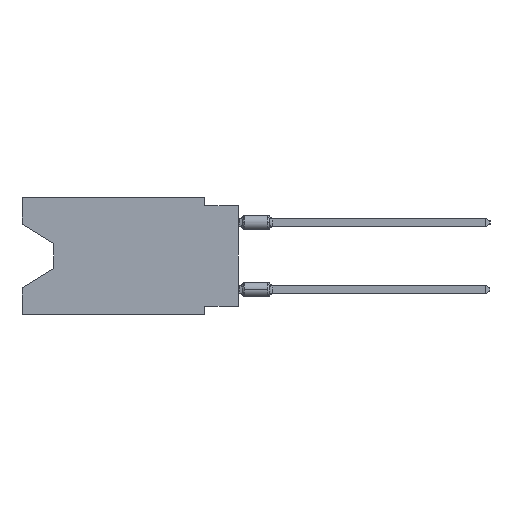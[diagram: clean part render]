
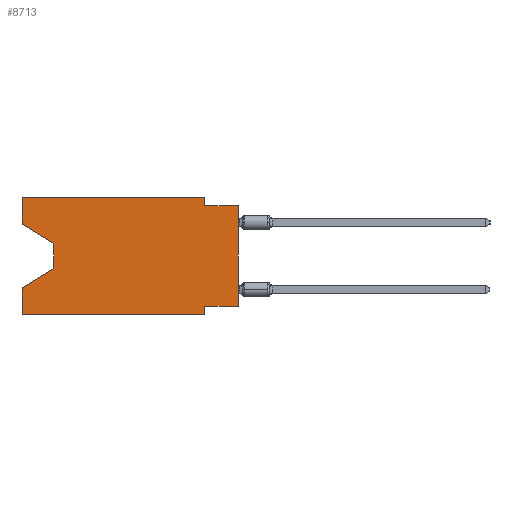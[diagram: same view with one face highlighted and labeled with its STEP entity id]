
A CAD part, left-side view. The second image highlights one B-rep face of the part: STEP entity #8713.
In plain terms, the highlighted planar face has unit normal (-1, 0, 0).
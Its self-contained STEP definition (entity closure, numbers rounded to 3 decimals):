
#262 = VECTOR ( 'NONE', #4472, 1000. ) ;
#289 = LINE ( 'NONE', #21041, #15894 ) ;
#421 = ORIENTED_EDGE ( 'NONE', *, *, #34585, .F. ) ;
#763 = EDGE_CURVE ( 'NONE', #27127, #10807, #26674, .T. ) ;
#1056 = DIRECTION ( 'NONE',  ( 0., -1., 0. ) ) ;
#1102 = CARTESIAN_POINT ( 'NONE',  ( 0., 16.383, -2.038 ) ) ;
#1876 = LINE ( 'NONE', #37017, #10331 ) ;
#2037 = LINE ( 'NONE', #4490, #2582 ) ;
#2582 = VECTOR ( 'NONE', #8059, 1000. ) ;
#3258 = VERTEX_POINT ( 'NONE', #36869 ) ;
#4444 = DIRECTION ( 'NONE',  ( 0., 0., 1. ) ) ;
#4472 = DIRECTION ( 'NONE',  ( 0., 0., -1. ) ) ;
#4490 = CARTESIAN_POINT ( 'NONE',  ( 0., 0., -0.635 ) ) ;
#5531 = CARTESIAN_POINT ( 'NONE',  ( 0., 16.383, -6.852 ) ) ;
#6348 = CARTESIAN_POINT ( 'NONE',  ( 0., 16.383, -8.89 ) ) ;
#6376 = DIRECTION ( 'NONE',  ( 1., 0., 0. ) ) ;
#7094 = LINE ( 'NONE', #15231, #14601 ) ;
#7292 = CARTESIAN_POINT ( 'NONE',  ( 0., 2.54, -8.89 ) ) ;
#7312 = CARTESIAN_POINT ( 'NONE',  ( 0., 13.97, -5.385 ) ) ;
#8059 = DIRECTION ( 'NONE',  ( 0., -1., 0. ) ) ;
#8412 = VERTEX_POINT ( 'NONE', #35254 ) ;
#8562 = VECTOR ( 'NONE', #34032, 1000. ) ;
#8713 = ADVANCED_FACE ( 'NONE', ( #29999 ), #35109, .F. ) ;
#9758 = DIRECTION ( 'NONE',  ( 0., 0., -1. ) ) ;
#9831 = VECTOR ( 'NONE', #27547, 1000. ) ;
#9863 = CARTESIAN_POINT ( 'NONE',  ( 0., 2.54, -8.89 ) ) ;
#10045 = ORIENTED_EDGE ( 'NONE', *, *, #763, .F. ) ;
#10190 = DIRECTION ( 'NONE',  ( 0., 0., 1. ) ) ;
#10331 = VECTOR ( 'NONE', #34185, 1000. ) ;
#10807 = VERTEX_POINT ( 'NONE', #35872 ) ;
#10969 = LINE ( 'NONE', #25162, #8562 ) ;
#11024 = VERTEX_POINT ( 'NONE', #36984 ) ;
#12344 = DIRECTION ( 'NONE',  ( 0., -1., 0. ) ) ;
#13097 = EDGE_CURVE ( 'NONE', #30204, #28272, #15877, .T. ) ;
#13838 = EDGE_CURVE ( 'NONE', #23940, #8412, #7094, .T. ) ;
#13853 = CARTESIAN_POINT ( 'NONE',  ( 0., 2.54, -8.255 ) ) ;
#14453 = CARTESIAN_POINT ( 'NONE',  ( 0., 0., -8.255 ) ) ;
#14601 = VECTOR ( 'NONE', #4444, 1000. ) ;
#15020 = EDGE_LOOP ( 'NONE', ( #34271, #21767, #30359, #18782, #26481, #421, #30838, #36578, #17789, #37287, #33578, #10045 ) ) ;
#15231 = CARTESIAN_POINT ( 'NONE',  ( 0., 0., 0. ) ) ;
#15499 = EDGE_CURVE ( 'NONE', #30204, #25587, #23366, .T. ) ;
#15877 = LINE ( 'NONE', #27414, #19702 ) ;
#15894 = VECTOR ( 'NONE', #12344, 1000. ) ;
#17789 = ORIENTED_EDGE ( 'NONE', *, *, #19752, .F. ) ;
#18639 = VECTOR ( 'NONE', #1056, 1000. ) ;
#18657 = CARTESIAN_POINT ( 'NONE',  ( 0., 16.383, -8.89 ) ) ;
#18782 = ORIENTED_EDGE ( 'NONE', *, *, #13097, .F. ) ;
#19695 = VERTEX_POINT ( 'NONE', #7312 ) ;
#19702 = VECTOR ( 'NONE', #10190, 1000. ) ;
#19752 = EDGE_CURVE ( 'NONE', #11024, #8412, #2037, .T. ) ;
#20224 = VERTEX_POINT ( 'NONE', #27878 ) ;
#20374 = EDGE_CURVE ( 'NONE', #10807, #20224, #289, .T. ) ;
#20463 = VECTOR ( 'NONE', #24564, 1000. ) ;
#21041 = CARTESIAN_POINT ( 'NONE',  ( 0., 16.383, 0. ) ) ;
#21767 = ORIENTED_EDGE ( 'NONE', *, *, #29984, .T. ) ;
#22931 = LINE ( 'NONE', #23496, #25750 ) ;
#23366 = LINE ( 'NONE', #6348, #18639 ) ;
#23496 = CARTESIAN_POINT ( 'NONE',  ( 0., 2.54, 0. ) ) ;
#23940 = VERTEX_POINT ( 'NONE', #14453 ) ;
#24007 = CARTESIAN_POINT ( 'NONE',  ( 0., 16.383, 0. ) ) ;
#24564 = DIRECTION ( 'NONE',  ( 0., 0., 1. ) ) ;
#25162 = CARTESIAN_POINT ( 'NONE',  ( 0., 13.97, -3.505 ) ) ;
#25458 = EDGE_CURVE ( 'NONE', #20224, #11024, #22931, .T. ) ;
#25587 = VERTEX_POINT ( 'NONE', #9863 ) ;
#25750 = VECTOR ( 'NONE', #34850, 1000. ) ;
#26481 = ORIENTED_EDGE ( 'NONE', *, *, #15499, .T. ) ;
#26627 = DIRECTION ( 'NONE',  ( 0., -0.855, -0.519 ) ) ;
#26674 = LINE ( 'NONE', #24007, #20463 ) ;
#26998 = LINE ( 'NONE', #1102, #36979 ) ;
#27127 = VERTEX_POINT ( 'NONE', #34210 ) ;
#27414 = CARTESIAN_POINT ( 'NONE',  ( 0., 16.383, 0. ) ) ;
#27547 = DIRECTION ( 'NONE',  ( 0., 1., 0. ) ) ;
#27878 = CARTESIAN_POINT ( 'NONE',  ( 0., 2.54, 0. ) ) ;
#28272 = VERTEX_POINT ( 'NONE', #5531 ) ;
#29258 = CARTESIAN_POINT ( 'NONE',  ( 0., 16.383, 0. ) ) ;
#29984 = EDGE_CURVE ( 'NONE', #3258, #19695, #10969, .T. ) ;
#29999 = FACE_OUTER_BOUND ( 'NONE', #15020, .T. ) ;
#30182 = LINE ( 'NONE', #7292, #262 ) ;
#30204 = VERTEX_POINT ( 'NONE', #18657 ) ;
#30359 = ORIENTED_EDGE ( 'NONE', *, *, #35945, .T. ) ;
#30838 = ORIENTED_EDGE ( 'NONE', *, *, #33703, .F. ) ;
#31153 = VERTEX_POINT ( 'NONE', #13853 ) ;
#33437 = AXIS2_PLACEMENT_3D ( 'NONE', #29258, #6376, #9758 ) ;
#33578 = ORIENTED_EDGE ( 'NONE', *, *, #20374, .F. ) ;
#33622 = EDGE_CURVE ( 'NONE', #27127, #3258, #26998, .T. ) ;
#33703 = EDGE_CURVE ( 'NONE', #23940, #31153, #36051, .T. ) ;
#34032 = DIRECTION ( 'NONE',  ( 0., 0., -1. ) ) ;
#34185 = DIRECTION ( 'NONE',  ( 0., 0.855, -0.519 ) ) ;
#34210 = CARTESIAN_POINT ( 'NONE',  ( 0., 16.383, -2.038 ) ) ;
#34271 = ORIENTED_EDGE ( 'NONE', *, *, #33622, .T. ) ;
#34585 = EDGE_CURVE ( 'NONE', #31153, #25587, #30182, .T. ) ;
#34850 = DIRECTION ( 'NONE',  ( 0., 0., -1. ) ) ;
#35109 = PLANE ( 'NONE',  #33437 ) ;
#35254 = CARTESIAN_POINT ( 'NONE',  ( 0., 0., -0.635 ) ) ;
#35872 = CARTESIAN_POINT ( 'NONE',  ( 0., 16.383, 0. ) ) ;
#35945 = EDGE_CURVE ( 'NONE', #19695, #28272, #1876, .T. ) ;
#36051 = LINE ( 'NONE', #36420, #9831 ) ;
#36420 = CARTESIAN_POINT ( 'NONE',  ( 0., 0., -8.255 ) ) ;
#36578 = ORIENTED_EDGE ( 'NONE', *, *, #13838, .T. ) ;
#36869 = CARTESIAN_POINT ( 'NONE',  ( 0., 13.97, -3.505 ) ) ;
#36979 = VECTOR ( 'NONE', #26627, 1000. ) ;
#36984 = CARTESIAN_POINT ( 'NONE',  ( 0., 2.54, -0.635 ) ) ;
#37017 = CARTESIAN_POINT ( 'NONE',  ( 0., 13.97, -5.385 ) ) ;
#37287 = ORIENTED_EDGE ( 'NONE', *, *, #25458, .F. ) ;
